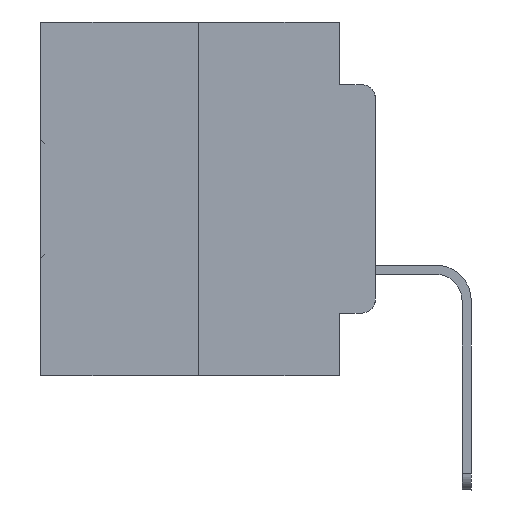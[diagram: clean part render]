
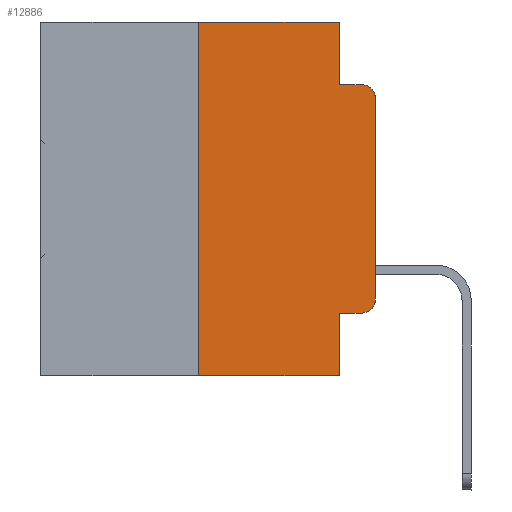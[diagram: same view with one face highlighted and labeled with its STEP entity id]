
A CAD part, left-side view. The second image highlights one B-rep face of the part: STEP entity #12886.
In plain terms, the highlighted planar face has unit normal (-1, 0, 0).
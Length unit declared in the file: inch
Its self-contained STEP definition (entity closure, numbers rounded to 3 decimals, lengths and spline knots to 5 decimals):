
#132 = VERTEX_POINT ( 'NONE', #10858 ) ;
#343 = LINE ( 'NONE', #2094, #10065 ) ;
#501 = DIRECTION ( 'NONE',  ( -1., 0., 0. ) ) ;
#553 = CARTESIAN_POINT ( 'NONE',  ( 0., 0., 0. ) ) ;
#825 = ORIENTED_EDGE ( 'NONE', *, *, #20032, .T. ) ;
#967 = ORIENTED_EDGE ( 'NONE', *, *, #1999, .T. ) ;
#1161 = LINE ( 'NONE', #24156, #13619 ) ;
#1290 = EDGE_CURVE ( 'NONE', #15818, #26275, #1161, .T. ) ;
#1999 = EDGE_CURVE ( 'NONE', #5986, #132, #17495, .T. ) ;
#2094 = CARTESIAN_POINT ( 'NONE',  ( 0., 0.25, 0. ) ) ;
#2255 = FACE_OUTER_BOUND ( 'NONE', #13474, .T. ) ;
#2264 = VECTOR ( 'NONE', #5193, 39.37008 ) ;
#2862 = VERTEX_POINT ( 'NONE', #13409 ) ;
#2894 = EDGE_CURVE ( 'NONE', #10198, #16793, #21758, .T. ) ;
#3003 = DIRECTION ( 'NONE',  ( 0., 0., -1. ) ) ;
#3063 = DIRECTION ( 'NONE',  ( 0., 0., 1. ) ) ;
#3864 = ORIENTED_EDGE ( 'NONE', *, *, #24247, .F. ) ;
#4414 = CARTESIAN_POINT ( 'NONE',  ( 0., 0.473, -0.5 ) ) ;
#4893 = CARTESIAN_POINT ( 'NONE',  ( 0., 0.051, 0. ) ) ;
#5193 = DIRECTION ( 'NONE',  ( 0., -1., 0. ) ) ;
#5770 = VECTOR ( 'NONE', #21220, 39.37008 ) ;
#5986 = VERTEX_POINT ( 'NONE', #26203 ) ;
#6545 = AXIS2_PLACEMENT_3D ( 'NONE', #6927, #24597, #22041 ) ;
#6927 = CARTESIAN_POINT ( 'NONE',  ( 0., 0.473, 0. ) ) ;
#7043 = DIRECTION ( 'NONE',  ( -1., 0., 0. ) ) ;
#8653 = ORIENTED_EDGE ( 'NONE', *, *, #2894, .T. ) ;
#8794 = VECTOR ( 'NONE', #20323, 39.37008 ) ;
#9424 = ORIENTED_EDGE ( 'NONE', *, *, #1290, .T. ) ;
#9549 = CIRCLE ( 'NONE', #25815, 0.02 ) ;
#10065 = VECTOR ( 'NONE', #19260, 39.37008 ) ;
#10198 = VERTEX_POINT ( 'NONE', #27189 ) ;
#10504 = VECTOR ( 'NONE', #19037, 39.37008 ) ;
#10858 = CARTESIAN_POINT ( 'NONE',  ( 0., 0.051, -0.5 ) ) ;
#11247 = LINE ( 'NONE', #30198, #2264 ) ;
#12245 = EDGE_CURVE ( 'NONE', #5986, #22082, #343, .T. ) ;
#12421 = CARTESIAN_POINT ( 'NONE',  ( 0., 0.051, -0.0885 ) ) ;
#12886 = ADVANCED_FACE ( 'NONE', ( #2255 ), #29959, .F. ) ;
#13030 = CARTESIAN_POINT ( 'NONE',  ( 0., 0.02, -0.1085 ) ) ;
#13409 = CARTESIAN_POINT ( 'NONE',  ( 0., 0.02, -0.0885 ) ) ;
#13428 = ORIENTED_EDGE ( 'NONE', *, *, #12245, .F. ) ;
#13474 = EDGE_LOOP ( 'NONE', ( #8653, #27707, #32420, #16045, #3864, #13428, #967, #15432, #9424, #825 ) ) ;
#13619 = VECTOR ( 'NONE', #21405, 39.37008 ) ;
#14171 = VERTEX_POINT ( 'NONE', #12421 ) ;
#14659 = CIRCLE ( 'NONE', #18385, 0.02 ) ;
#15432 = ORIENTED_EDGE ( 'NONE', *, *, #19512, .F. ) ;
#15818 = VERTEX_POINT ( 'NONE', #21037 ) ;
#16045 = ORIENTED_EDGE ( 'NONE', *, *, #23880, .F. ) ;
#16480 = CARTESIAN_POINT ( 'NONE',  ( 0., 0.051, 0. ) ) ;
#16793 = VERTEX_POINT ( 'NONE', #22845 ) ;
#17125 = CARTESIAN_POINT ( 'NONE',  ( 0., 0.25, 0. ) ) ;
#17188 = DIRECTION ( 'NONE',  ( 0., -1., 0. ) ) ;
#17495 = LINE ( 'NONE', #4414, #18279 ) ;
#18279 = VECTOR ( 'NONE', #17188, 39.37008 ) ;
#18385 = AXIS2_PLACEMENT_3D ( 'NONE', #13030, #501, #3003 ) ;
#18462 = EDGE_CURVE ( 'NONE', #16793, #2862, #14659, .T. ) ;
#19037 = DIRECTION ( 'NONE',  ( 0., -1., 0. ) ) ;
#19116 = LINE ( 'NONE', #16480, #5770 ) ;
#19260 = DIRECTION ( 'NONE',  ( 0., 0., 1. ) ) ;
#19512 = EDGE_CURVE ( 'NONE', #15818, #132, #24532, .T. ) ;
#19818 = VECTOR ( 'NONE', #3063, 39.37008 ) ;
#20032 = EDGE_CURVE ( 'NONE', #26275, #10198, #9549, .T. ) ;
#20323 = DIRECTION ( 'NONE',  ( 0., 0., -1. ) ) ;
#21037 = CARTESIAN_POINT ( 'NONE',  ( 0., 0.051, -0.4115 ) ) ;
#21220 = DIRECTION ( 'NONE',  ( 0., 0., -1. ) ) ;
#21405 = DIRECTION ( 'NONE',  ( 0., -1., 0. ) ) ;
#21758 = LINE ( 'NONE', #553, #19818 ) ;
#22041 = DIRECTION ( 'NONE',  ( 0., 0., -1. ) ) ;
#22082 = VERTEX_POINT ( 'NONE', #17125 ) ;
#22693 = CARTESIAN_POINT ( 'NONE',  ( 0., 0.051, 0. ) ) ;
#22845 = CARTESIAN_POINT ( 'NONE',  ( 0., 0., -0.1085 ) ) ;
#23880 = EDGE_CURVE ( 'NONE', #24688, #14171, #19116, .T. ) ;
#24156 = CARTESIAN_POINT ( 'NONE',  ( 0., 0.051, -0.4115 ) ) ;
#24247 = EDGE_CURVE ( 'NONE', #22082, #24688, #11247, .T. ) ;
#24306 = CARTESIAN_POINT ( 'NONE',  ( 0., 0.051, -0.0885 ) ) ;
#24532 = LINE ( 'NONE', #4893, #8794 ) ;
#24597 = DIRECTION ( 'NONE',  ( 1., 0., 0. ) ) ;
#24601 = DIRECTION ( 'NONE',  ( 0., 0., -1. ) ) ;
#24688 = VERTEX_POINT ( 'NONE', #22693 ) ;
#24920 = CARTESIAN_POINT ( 'NONE',  ( 0., 0.02, -0.3915 ) ) ;
#25815 = AXIS2_PLACEMENT_3D ( 'NONE', #24920, #7043, #24601 ) ;
#26203 = CARTESIAN_POINT ( 'NONE',  ( 0., 0.25, -0.5 ) ) ;
#26275 = VERTEX_POINT ( 'NONE', #28666 ) ;
#27189 = CARTESIAN_POINT ( 'NONE',  ( 0., 0., -0.3915 ) ) ;
#27707 = ORIENTED_EDGE ( 'NONE', *, *, #18462, .T. ) ;
#28246 = EDGE_CURVE ( 'NONE', #14171, #2862, #32134, .T. ) ;
#28666 = CARTESIAN_POINT ( 'NONE',  ( 0., 0.02, -0.4115 ) ) ;
#29959 = PLANE ( 'NONE',  #6545 ) ;
#30198 = CARTESIAN_POINT ( 'NONE',  ( 0., 0.473, 0. ) ) ;
#32134 = LINE ( 'NONE', #24306, #10504 ) ;
#32420 = ORIENTED_EDGE ( 'NONE', *, *, #28246, .F. ) ;
